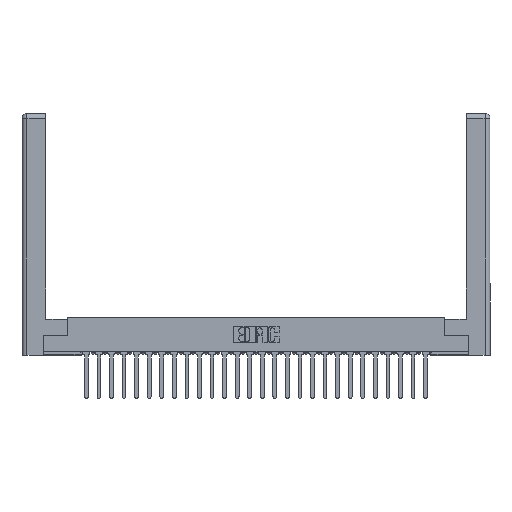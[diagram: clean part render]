
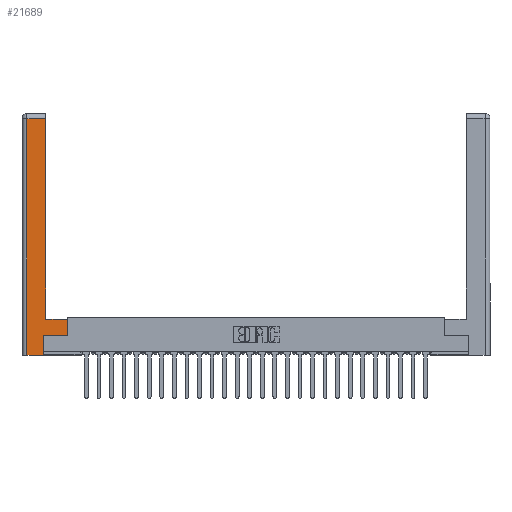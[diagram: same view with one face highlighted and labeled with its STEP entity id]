
A CAD part, top view. The second image highlights one B-rep face of the part: STEP entity #21689.
In plain terms, the highlighted planar face has unit normal (0, 0, 1).
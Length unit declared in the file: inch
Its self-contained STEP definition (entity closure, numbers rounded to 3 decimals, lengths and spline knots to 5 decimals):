
#182 = ORIENTED_EDGE ( 'NONE', *, *, #14162, .T. ) ;
#747 = VERTEX_POINT ( 'NONE', #24061 ) ;
#949 = CARTESIAN_POINT ( 'NONE',  ( 0.565, 0.45, 0. ) ) ;
#1129 = CARTESIAN_POINT ( 'NONE',  ( 0.265, 0.245, 0. ) ) ;
#1384 = DIRECTION ( 'NONE',  ( 1., 0., 0. ) ) ;
#1553 = CARTESIAN_POINT ( 'NONE',  ( 0.0615, 0., 0. ) ) ;
#1596 = VERTEX_POINT ( 'NONE', #949 ) ;
#2866 = CARTESIAN_POINT ( 'NONE',  ( 0.0615, 2.94, 0. ) ) ;
#2902 = CARTESIAN_POINT ( 'NONE',  ( 0.295, 0.45, 0. ) ) ;
#3314 = LINE ( 'NONE', #19533, #8423 ) ;
#3745 = FACE_OUTER_BOUND ( 'NONE', #25299, .T. ) ;
#4085 = LINE ( 'NONE', #24517, #15784 ) ;
#4719 = VECTOR ( 'NONE', #16808, 39.37008 ) ;
#4876 = CARTESIAN_POINT ( 'NONE',  ( 0.295, 2.94, 0. ) ) ;
#5730 = DIRECTION ( 'NONE',  ( 0., 1., 0. ) ) ;
#6012 = DIRECTION ( 'NONE',  ( 1., 0., 0. ) ) ;
#6207 = VECTOR ( 'NONE', #11898, 39.37008 ) ;
#6646 = CARTESIAN_POINT ( 'NONE',  ( 0., 0., 0. ) ) ;
#8136 = VERTEX_POINT ( 'NONE', #4876 ) ;
#8423 = VECTOR ( 'NONE', #17517, 39.37008 ) ;
#8477 = ORIENTED_EDGE ( 'NONE', *, *, #24702, .T. ) ;
#8617 = DIRECTION ( 'NONE',  ( -1., 0., 0. ) ) ;
#9275 = LINE ( 'NONE', #2866, #6207 ) ;
#9281 = AXIS2_PLACEMENT_3D ( 'NONE', #6646, #15705, #13399 ) ;
#9436 = LINE ( 'NONE', #27762, #13957 ) ;
#11671 = EDGE_CURVE ( 'NONE', #28016, #20244, #17887, .T. ) ;
#11898 = DIRECTION ( 'NONE',  ( -1., 0., 0. ) ) ;
#12002 = VERTEX_POINT ( 'NONE', #2902 ) ;
#12576 = CARTESIAN_POINT ( 'NONE',  ( 0.265, 0.245, 0. ) ) ;
#12830 = ORIENTED_EDGE ( 'NONE', *, *, #19563, .T. ) ;
#13399 = DIRECTION ( 'NONE',  ( -1., 0., 0. ) ) ;
#13648 = EDGE_CURVE ( 'NONE', #1596, #12002, #16740, .T. ) ;
#13957 = VECTOR ( 'NONE', #6012, 39.37008 ) ;
#14162 = EDGE_CURVE ( 'NONE', #22526, #747, #9436, .T. ) ;
#14514 = CARTESIAN_POINT ( 'NONE',  ( 0.565, 0.245, 0. ) ) ;
#15105 = CARTESIAN_POINT ( 'NONE',  ( 0.565, 0.245, 0. ) ) ;
#15353 = EDGE_CURVE ( 'NONE', #8136, #25370, #9275, .T. ) ;
#15391 = CARTESIAN_POINT ( 'NONE',  ( 0.295, 0.45, 0. ) ) ;
#15705 = DIRECTION ( 'NONE',  ( 0., 0., -1. ) ) ;
#15784 = VECTOR ( 'NONE', #24336, 39.37008 ) ;
#16410 = LINE ( 'NONE', #27679, #4719 ) ;
#16740 = LINE ( 'NONE', #15391, #17060 ) ;
#16808 = DIRECTION ( 'NONE',  ( 0., 1., 0. ) ) ;
#17060 = VECTOR ( 'NONE', #8617, 39.37008 ) ;
#17517 = DIRECTION ( 'NONE',  ( 0., -1., 0. ) ) ;
#17618 = PLANE ( 'NONE',  #9281 ) ;
#17887 = LINE ( 'NONE', #14514, #24039 ) ;
#19533 = CARTESIAN_POINT ( 'NONE',  ( 0.0615, 0., 0. ) ) ;
#19563 = EDGE_CURVE ( 'NONE', #25370, #22526, #3314, .T. ) ;
#20090 = ORIENTED_EDGE ( 'NONE', *, *, #15353, .T. ) ;
#20230 = ORIENTED_EDGE ( 'NONE', *, *, #22447, .T. ) ;
#20244 = VERTEX_POINT ( 'NONE', #15105 ) ;
#20283 = CARTESIAN_POINT ( 'NONE',  ( 0.0615, 2.94, 0. ) ) ;
#21689 = ADVANCED_FACE ( 'NONE', ( #3745 ), #17618, .F. ) ;
#22447 = EDGE_CURVE ( 'NONE', #20244, #1596, #16410, .T. ) ;
#22526 = VERTEX_POINT ( 'NONE', #1553 ) ;
#23467 = VECTOR ( 'NONE', #5730, 39.37008 ) ;
#24039 = VECTOR ( 'NONE', #1384, 39.37008 ) ;
#24061 = CARTESIAN_POINT ( 'NONE',  ( 0.265, 0., 0. ) ) ;
#24336 = DIRECTION ( 'NONE',  ( 0., 1., 0. ) ) ;
#24517 = CARTESIAN_POINT ( 'NONE',  ( 0.295, 3., 0. ) ) ;
#24638 = ORIENTED_EDGE ( 'NONE', *, *, #11671, .T. ) ;
#24702 = EDGE_CURVE ( 'NONE', #12002, #8136, #4085, .T. ) ;
#24765 = ORIENTED_EDGE ( 'NONE', *, *, #26261, .T. ) ;
#25299 = EDGE_LOOP ( 'NONE', ( #8477, #20090, #12830, #182, #24765, #24638, #20230, #25589 ) ) ;
#25370 = VERTEX_POINT ( 'NONE', #20283 ) ;
#25589 = ORIENTED_EDGE ( 'NONE', *, *, #13648, .T. ) ;
#26261 = EDGE_CURVE ( 'NONE', #747, #28016, #27537, .T. ) ;
#27537 = LINE ( 'NONE', #12576, #23467 ) ;
#27679 = CARTESIAN_POINT ( 'NONE',  ( 0.565, 0.45, 0. ) ) ;
#27762 = CARTESIAN_POINT ( 'NONE',  ( 0.265, 0., 0. ) ) ;
#28016 = VERTEX_POINT ( 'NONE', #1129 ) ;
